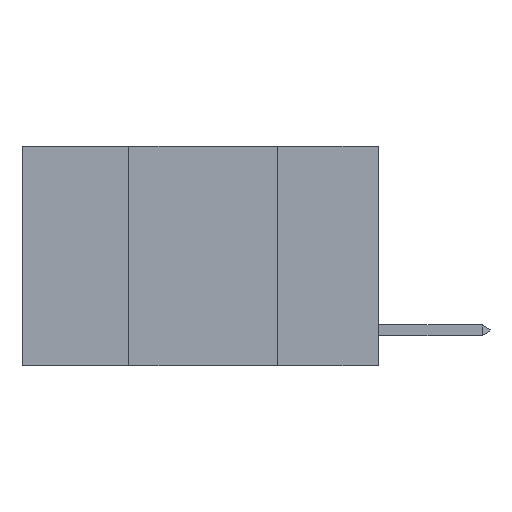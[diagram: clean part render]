
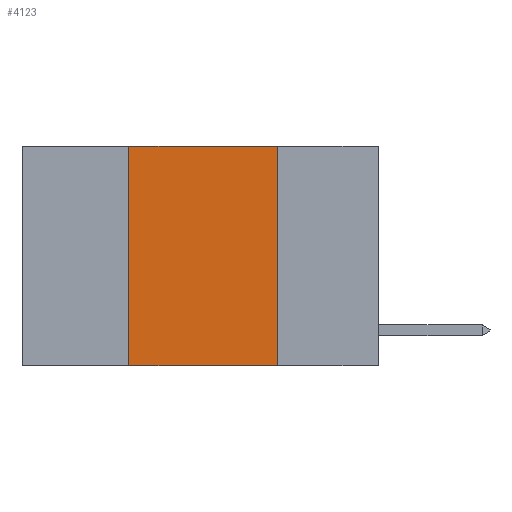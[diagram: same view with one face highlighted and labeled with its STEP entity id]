
A CAD part, left-side view. The second image highlights one B-rep face of the part: STEP entity #4123.
In plain terms, the highlighted planar face has unit normal (-1, 0, 0).
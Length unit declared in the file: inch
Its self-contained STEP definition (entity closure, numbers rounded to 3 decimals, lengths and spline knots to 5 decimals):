
#39 = DIRECTION ( 'NONE',  ( 0., -1., 0. ) ) ;
#108 = ORIENTED_EDGE ( 'NONE', *, *, #8219, .F. ) ;
#201 = CARTESIAN_POINT ( 'NONE',  ( 0., 0.42, 0. ) ) ;
#299 = DIRECTION ( 'NONE',  ( 0., 0., 1. ) ) ;
#367 = VERTEX_POINT ( 'NONE', #2876 ) ;
#416 = PLANE ( 'NONE',  #7785 ) ;
#750 = VECTOR ( 'NONE', #3851, 39.37008 ) ;
#858 = VERTEX_POINT ( 'NONE', #5152 ) ;
#935 = EDGE_LOOP ( 'NONE', ( #108, #1200, #7043, #9247 ) ) ;
#1200 = ORIENTED_EDGE ( 'NONE', *, *, #6495, .F. ) ;
#1369 = VERTEX_POINT ( 'NONE', #7098 ) ;
#1470 = VECTOR ( 'NONE', #299, 39.37008 ) ;
#1759 = LINE ( 'NONE', #201, #1470 ) ;
#1795 = VECTOR ( 'NONE', #39, 39.37008 ) ;
#1861 = CARTESIAN_POINT ( 'NONE',  ( 0., 0.17, -0.37 ) ) ;
#2816 = CARTESIAN_POINT ( 'NONE',  ( 0., 0.6, 0. ) ) ;
#2876 = CARTESIAN_POINT ( 'NONE',  ( 0., 0.17, 0. ) ) ;
#3517 = DIRECTION ( 'NONE',  ( 0., 0., -1. ) ) ;
#3525 = CARTESIAN_POINT ( 'NONE',  ( 0., 0.6, -0.37 ) ) ;
#3814 = VERTEX_POINT ( 'NONE', #1861 ) ;
#3851 = DIRECTION ( 'NONE',  ( 0., 0., -1. ) ) ;
#4123 = ADVANCED_FACE ( 'NONE', ( #6866 ), #416, .F. ) ;
#4128 = DIRECTION ( 'NONE',  ( 1., 0., 0. ) ) ;
#4513 = CARTESIAN_POINT ( 'NONE',  ( 0., 0.17, 0. ) ) ;
#5041 = DIRECTION ( 'NONE',  ( 0., -1., 0. ) ) ;
#5152 = CARTESIAN_POINT ( 'NONE',  ( 0., 0.42, -0.37 ) ) ;
#6282 = LINE ( 'NONE', #3525, #1795 ) ;
#6401 = CARTESIAN_POINT ( 'NONE',  ( 0., 0.6, 0. ) ) ;
#6484 = EDGE_CURVE ( 'NONE', #858, #3814, #6282, .T. ) ;
#6495 = EDGE_CURVE ( 'NONE', #1369, #367, #9242, .T. ) ;
#6866 = FACE_OUTER_BOUND ( 'NONE', #935, .T. ) ;
#7043 = ORIENTED_EDGE ( 'NONE', *, *, #7207, .F. ) ;
#7047 = VECTOR ( 'NONE', #5041, 39.37008 ) ;
#7098 = CARTESIAN_POINT ( 'NONE',  ( 0., 0.42, 0. ) ) ;
#7207 = EDGE_CURVE ( 'NONE', #858, #1369, #1759, .T. ) ;
#7296 = LINE ( 'NONE', #4513, #750 ) ;
#7785 = AXIS2_PLACEMENT_3D ( 'NONE', #6401, #4128, #3517 ) ;
#8219 = EDGE_CURVE ( 'NONE', #367, #3814, #7296, .T. ) ;
#9242 = LINE ( 'NONE', #2816, #7047 ) ;
#9247 = ORIENTED_EDGE ( 'NONE', *, *, #6484, .T. ) ;
